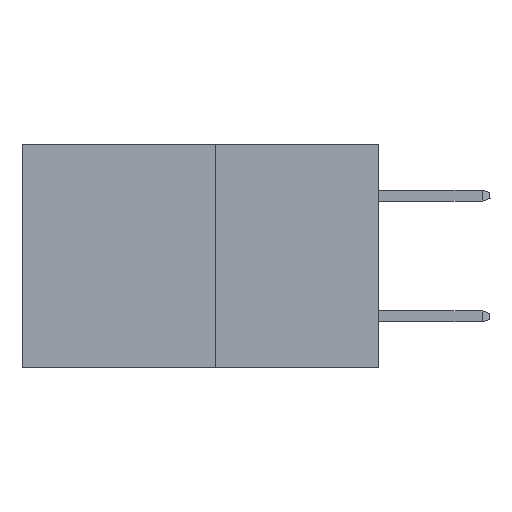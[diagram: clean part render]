
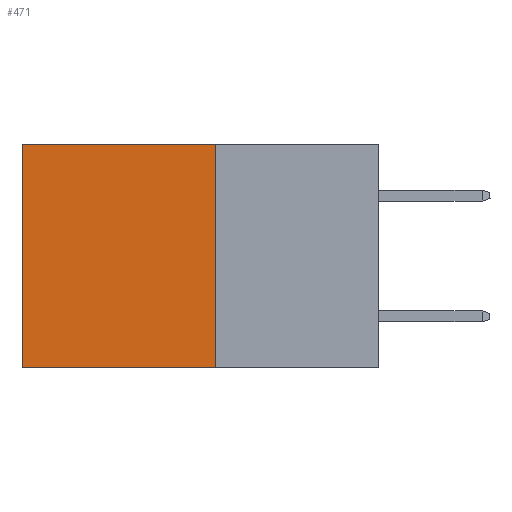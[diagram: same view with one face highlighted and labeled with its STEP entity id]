
A CAD part, left-side view. The second image highlights one B-rep face of the part: STEP entity #471.
In plain terms, the highlighted planar face has unit normal (-1, 0, 0).
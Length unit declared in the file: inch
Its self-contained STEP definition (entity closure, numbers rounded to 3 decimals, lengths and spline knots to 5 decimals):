
#312 = CARTESIAN_POINT ( 'NONE',  ( 0.277, 0.59, -0.37 ) ) ;
#375 = ORIENTED_EDGE ( 'NONE', *, *, #8053, .T. ) ;
#444 = ORIENTED_EDGE ( 'NONE', *, *, #5413, .F. ) ;
#454 = DIRECTION ( 'NONE',  ( 0., 1., 0. ) ) ;
#471 = ADVANCED_FACE ( 'NONE', ( #3021 ), #12693, .F. ) ;
#1473 = VECTOR ( 'NONE', #454, 39.37008 ) ;
#1633 = CARTESIAN_POINT ( 'NONE',  ( 0.277, 0.59, -0.37 ) ) ;
#2779 = CARTESIAN_POINT ( 'NONE',  ( 0.277, 0.27, -0.37 ) ) ;
#2859 = CARTESIAN_POINT ( 'NONE',  ( 0.277, 0.27, -0.37 ) ) ;
#3021 = FACE_OUTER_BOUND ( 'NONE', #11528, .T. ) ;
#3054 = LINE ( 'NONE', #1633, #11663 ) ;
#3319 = DIRECTION ( 'NONE',  ( 0., 0., -1. ) ) ;
#4553 = LINE ( 'NONE', #2859, #1473 ) ;
#5413 = EDGE_CURVE ( 'NONE', #10684, #9403, #5621, .T. ) ;
#5512 = VERTEX_POINT ( 'NONE', #13689 ) ;
#5621 = LINE ( 'NONE', #2779, #14655 ) ;
#7024 = VECTOR ( 'NONE', #10027, 39.37008 ) ;
#7072 = AXIS2_PLACEMENT_3D ( 'NONE', #14406, #8007, #3319 ) ;
#7155 = ORIENTED_EDGE ( 'NONE', *, *, #10632, .F. ) ;
#7377 = EDGE_CURVE ( 'NONE', #5512, #8468, #3054, .T. ) ;
#7405 = LINE ( 'NONE', #10077, #7024 ) ;
#8007 = DIRECTION ( 'NONE',  ( 1., 0., 0. ) ) ;
#8053 = EDGE_CURVE ( 'NONE', #10684, #5512, #7405, .T. ) ;
#8468 = VERTEX_POINT ( 'NONE', #312 ) ;
#9403 = VERTEX_POINT ( 'NONE', #12241 ) ;
#10027 = DIRECTION ( 'NONE',  ( 0., 1., 0. ) ) ;
#10077 = CARTESIAN_POINT ( 'NONE',  ( 0.277, 0.27, 0. ) ) ;
#10632 = EDGE_CURVE ( 'NONE', #9403, #8468, #4553, .T. ) ;
#10684 = VERTEX_POINT ( 'NONE', #14646 ) ;
#11528 = EDGE_LOOP ( 'NONE', ( #15213, #7155, #444, #375 ) ) ;
#11663 = VECTOR ( 'NONE', #14023, 39.37008 ) ;
#12241 = CARTESIAN_POINT ( 'NONE',  ( 0.277, 0.27, -0.37 ) ) ;
#12673 = DIRECTION ( 'NONE',  ( 0., 0., -1. ) ) ;
#12693 = PLANE ( 'NONE',  #7072 ) ;
#13689 = CARTESIAN_POINT ( 'NONE',  ( 0.277, 0.59, 0. ) ) ;
#14023 = DIRECTION ( 'NONE',  ( 0., 0., -1. ) ) ;
#14406 = CARTESIAN_POINT ( 'NONE',  ( 0.277, 0.27, -0.37 ) ) ;
#14646 = CARTESIAN_POINT ( 'NONE',  ( 0.277, 0.27, 0. ) ) ;
#14655 = VECTOR ( 'NONE', #12673, 39.37008 ) ;
#15213 = ORIENTED_EDGE ( 'NONE', *, *, #7377, .T. ) ;
